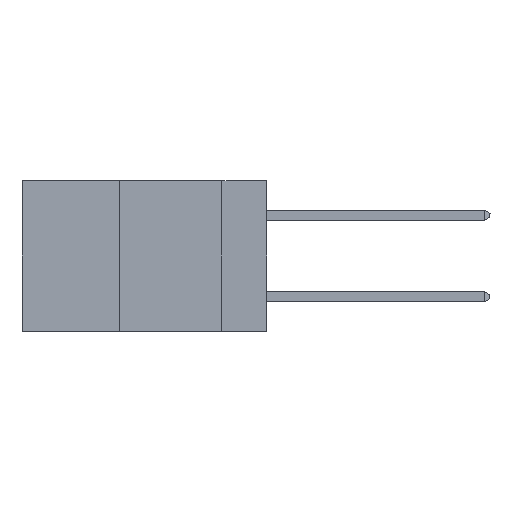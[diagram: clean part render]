
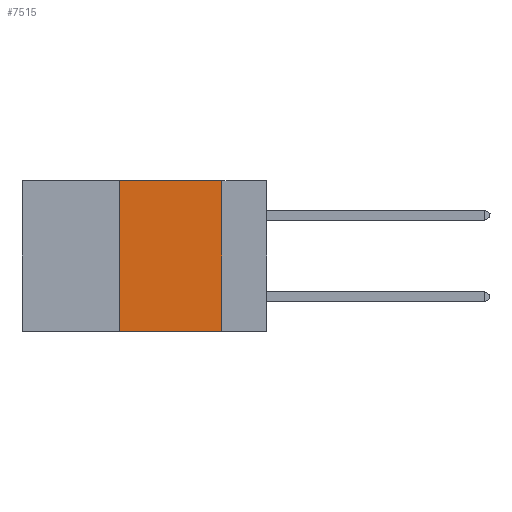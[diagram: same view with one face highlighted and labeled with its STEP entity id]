
A CAD part, left-side view. The second image highlights one B-rep face of the part: STEP entity #7515.
In plain terms, the highlighted planar face has unit normal (-1, 0, 0).
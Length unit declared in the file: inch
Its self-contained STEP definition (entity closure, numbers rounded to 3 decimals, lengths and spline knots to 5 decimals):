
#1127 = DIRECTION ( 'NONE',  ( 0., 0., -1. ) ) ;
#1502 = EDGE_CURVE ( 'NONE', #16155, #13228, #19976, .T. ) ;
#3137 = VECTOR ( 'NONE', #32100, 39.37008 ) ;
#5432 = VERTEX_POINT ( 'NONE', #30934 ) ;
#7515 = ADVANCED_FACE ( 'NONE', ( #24275 ), #36041, .F. ) ;
#8236 = ORIENTED_EDGE ( 'NONE', *, *, #9554, .F. ) ;
#8766 = EDGE_CURVE ( 'NONE', #16155, #19613, #12907, .T. ) ;
#9554 = EDGE_CURVE ( 'NONE', #5432, #13228, #37521, .T. ) ;
#11852 = DIRECTION ( 'NONE',  ( 0., -1., 0. ) ) ;
#12619 = CARTESIAN_POINT ( 'NONE',  ( 0., 0.36, -0.37 ) ) ;
#12907 = LINE ( 'NONE', #32976, #16266 ) ;
#13079 = EDGE_LOOP ( 'NONE', ( #8236, #36495, #26957, #24233 ) ) ;
#13143 = CARTESIAN_POINT ( 'NONE',  ( 0., 0.36, 0. ) ) ;
#13228 = VERTEX_POINT ( 'NONE', #29203 ) ;
#14370 = DIRECTION ( 'NONE',  ( 0., 0., -1. ) ) ;
#15531 = VECTOR ( 'NONE', #11852, 39.37008 ) ;
#16155 = VERTEX_POINT ( 'NONE', #12619 ) ;
#16266 = VECTOR ( 'NONE', #21017, 39.37008 ) ;
#17261 = CARTESIAN_POINT ( 'NONE',  ( 0., 0.6, 0. ) ) ;
#19613 = VERTEX_POINT ( 'NONE', #13143 ) ;
#19976 = LINE ( 'NONE', #28847, #15531 ) ;
#21017 = DIRECTION ( 'NONE',  ( 0., 0., 1. ) ) ;
#21388 = CARTESIAN_POINT ( 'NONE',  ( 0., 0.6, 0. ) ) ;
#24233 = ORIENTED_EDGE ( 'NONE', *, *, #1502, .T. ) ;
#24275 = FACE_OUTER_BOUND ( 'NONE', #13079, .T. ) ;
#26697 = LINE ( 'NONE', #17261, #3137 ) ;
#26957 = ORIENTED_EDGE ( 'NONE', *, *, #8766, .F. ) ;
#27849 = AXIS2_PLACEMENT_3D ( 'NONE', #21388, #32965, #1127 ) ;
#28847 = CARTESIAN_POINT ( 'NONE',  ( 0., 0.6, -0.37 ) ) ;
#29203 = CARTESIAN_POINT ( 'NONE',  ( 0., 0.11, -0.37 ) ) ;
#30934 = CARTESIAN_POINT ( 'NONE',  ( 0., 0.11, 0. ) ) ;
#32100 = DIRECTION ( 'NONE',  ( 0., -1., 0. ) ) ;
#32826 = VECTOR ( 'NONE', #14370, 39.37008 ) ;
#32965 = DIRECTION ( 'NONE',  ( 1., 0., 0. ) ) ;
#32976 = CARTESIAN_POINT ( 'NONE',  ( 0., 0.36, 0. ) ) ;
#33521 = EDGE_CURVE ( 'NONE', #19613, #5432, #26697, .T. ) ;
#36041 = PLANE ( 'NONE',  #27849 ) ;
#36495 = ORIENTED_EDGE ( 'NONE', *, *, #33521, .F. ) ;
#37521 = LINE ( 'NONE', #37699, #32826 ) ;
#37699 = CARTESIAN_POINT ( 'NONE',  ( 0., 0.11, 0. ) ) ;
